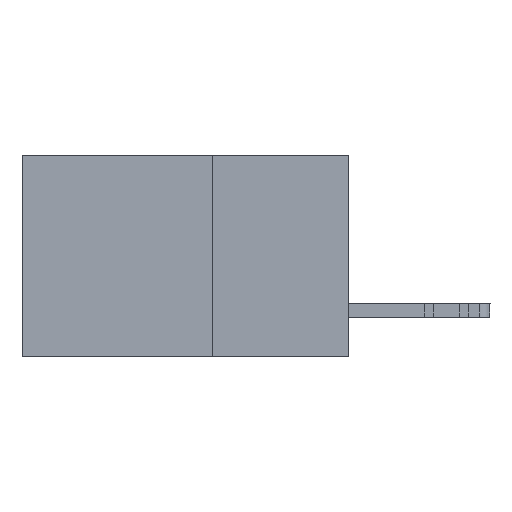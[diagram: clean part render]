
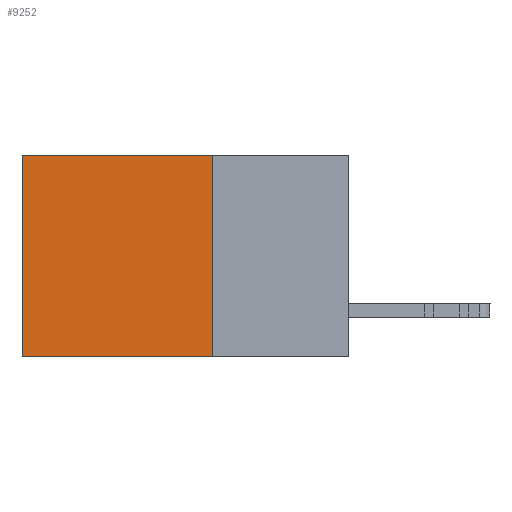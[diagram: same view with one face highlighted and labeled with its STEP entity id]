
A CAD part, left-side view. The second image highlights one B-rep face of the part: STEP entity #9252.
In plain terms, the highlighted planar face has unit normal (-1, 0, 0).
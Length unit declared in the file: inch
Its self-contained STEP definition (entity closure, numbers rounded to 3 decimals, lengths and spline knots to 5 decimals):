
#598 = VECTOR ( 'NONE', #8802, 39.37008 ) ;
#646 = VECTOR ( 'NONE', #10339, 39.37008 ) ;
#1259 = CARTESIAN_POINT ( 'NONE',  ( 0.2615, 0.25, 0. ) ) ;
#1462 = EDGE_CURVE ( 'NONE', #10194, #22775, #18027, .T. ) ;
#1494 = LINE ( 'NONE', #1259, #598 ) ;
#1783 = CARTESIAN_POINT ( 'NONE',  ( 0.2615, 0.6, -0.37 ) ) ;
#2232 = DIRECTION ( 'NONE',  ( 0., 0., -1. ) ) ;
#2543 = VERTEX_POINT ( 'NONE', #11389 ) ;
#3210 = PLANE ( 'NONE',  #22573 ) ;
#3399 = VERTEX_POINT ( 'NONE', #1783 ) ;
#4905 = ORIENTED_EDGE ( 'NONE', *, *, #22028, .T. ) ;
#7130 = ORIENTED_EDGE ( 'NONE', *, *, #23106, .F. ) ;
#7385 = EDGE_LOOP ( 'NONE', ( #4905, #7130, #14586, #13391 ) ) ;
#7791 = CARTESIAN_POINT ( 'NONE',  ( 0.2615, 0.25, -0.37 ) ) ;
#8123 = VECTOR ( 'NONE', #2232, 39.37008 ) ;
#8263 = DIRECTION ( 'NONE',  ( 0., 0., -1. ) ) ;
#8802 = DIRECTION ( 'NONE',  ( 0., 1., 0. ) ) ;
#9252 = ADVANCED_FACE ( 'NONE', ( #14464 ), #3210, .F. ) ;
#9339 = DIRECTION ( 'NONE',  ( 0., 0., -1. ) ) ;
#10194 = VERTEX_POINT ( 'NONE', #16367 ) ;
#10339 = DIRECTION ( 'NONE',  ( 0., 1., 0. ) ) ;
#10740 = CARTESIAN_POINT ( 'NONE',  ( 0.2615, 0.25, -0.37 ) ) ;
#11389 = CARTESIAN_POINT ( 'NONE',  ( 0.2615, 0.6, 0. ) ) ;
#11618 = CARTESIAN_POINT ( 'NONE',  ( 0.2615, 0.6, -0.37 ) ) ;
#12312 = CARTESIAN_POINT ( 'NONE',  ( 0.2615, 0.25, -0.37 ) ) ;
#13391 = ORIENTED_EDGE ( 'NONE', *, *, #22156, .T. ) ;
#14464 = FACE_OUTER_BOUND ( 'NONE', #7385, .T. ) ;
#14586 = ORIENTED_EDGE ( 'NONE', *, *, #1462, .F. ) ;
#16367 = CARTESIAN_POINT ( 'NONE',  ( 0.2615, 0.25, 0. ) ) ;
#18027 = LINE ( 'NONE', #12312, #21724 ) ;
#18865 = DIRECTION ( 'NONE',  ( 1., 0., 0. ) ) ;
#21029 = LINE ( 'NONE', #11618, #8123 ) ;
#21497 = CARTESIAN_POINT ( 'NONE',  ( 0.2615, 0.25, -0.37 ) ) ;
#21724 = VECTOR ( 'NONE', #8263, 39.37008 ) ;
#22028 = EDGE_CURVE ( 'NONE', #2543, #3399, #21029, .T. ) ;
#22156 = EDGE_CURVE ( 'NONE', #10194, #2543, #1494, .T. ) ;
#22573 = AXIS2_PLACEMENT_3D ( 'NONE', #10740, #18865, #9339 ) ;
#22775 = VERTEX_POINT ( 'NONE', #7791 ) ;
#23106 = EDGE_CURVE ( 'NONE', #22775, #3399, #23328, .T. ) ;
#23328 = LINE ( 'NONE', #21497, #646 ) ;
